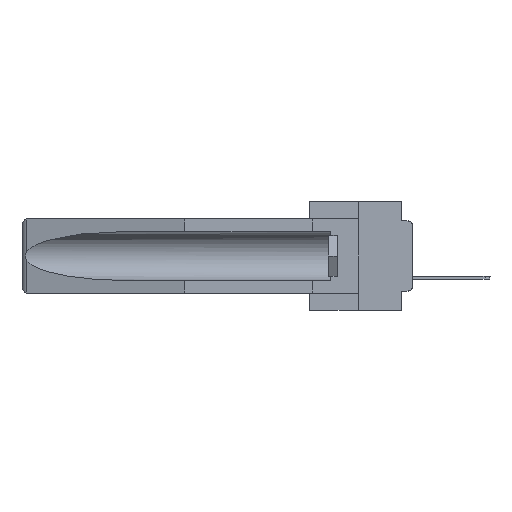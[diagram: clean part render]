
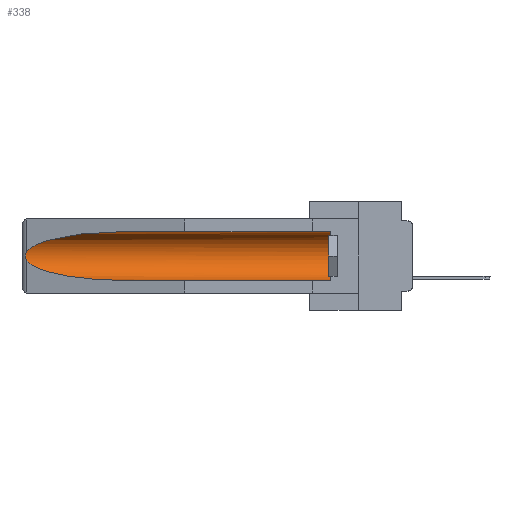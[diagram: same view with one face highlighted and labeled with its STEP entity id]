
A CAD part, left-side view. The second image highlights one B-rep face of the part: STEP entity #338.
In plain terms, the highlighted cylindrical face has radius 2.857 mm (diameter 5.715 mm), a partial arc.
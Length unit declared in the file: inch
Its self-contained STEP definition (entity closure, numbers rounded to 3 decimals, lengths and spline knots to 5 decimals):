
#177 = ORIENTED_EDGE ( 'NONE', *, *, #3073, .T. ) ;
#234 = CARTESIAN_POINT ( 'NONE',  ( 0.155, 1.07973, -0.059 ) ) ;
#338 = ADVANCED_FACE ( 'NONE', ( #30884 ), #16875, .F. ) ;
#2537 = CARTESIAN_POINT ( 'NONE',  ( 0.155, -0.30754, -0.1715 ) ) ;
#3073 = EDGE_CURVE ( 'NONE', #8887, #26737, #36057, .T. ) ;
#3840 = CARTESIAN_POINT ( 'NONE',  ( 0.25451, 1.48313, -0.09465 ) ) ;
#4493 = DIRECTION ( 'NONE',  ( 0., -1., 0. ) ) ;
#5424 = VERTEX_POINT ( 'NONE', #23797 ) ;
#6087 = ORIENTED_EDGE ( 'NONE', *, *, #17450, .T. ) ;
#6566 = CARTESIAN_POINT ( 'NONE',  ( 0.155, -0.30754, -0.284 ) ) ;
#6943 = DIRECTION ( 'NONE',  ( 0., 0., 1. ) ) ;
#6955 = AXIS2_PLACEMENT_3D ( 'NONE', #2537, #21308, #15341 ) ;
#8093 = CARTESIAN_POINT ( 'NONE',  ( 0.25451, 1.48313, -0.24835 ) ) ;
#8133 = AXIS2_PLACEMENT_3D ( 'NONE', #20806, #4493, #6943 ) ;
#8412 = CARTESIAN_POINT ( 'NONE',  ( 0.2673, 1.5327, -0.16383 ) ) ;
#8449 = CARTESIAN_POINT ( 'NONE',  ( 0.155, 1.07973, -0.284 ) ) ;
#8887 = VERTEX_POINT ( 'NONE', #15467 ) ;
#9172 = ORIENTED_EDGE ( 'NONE', *, *, #31409, .T. ) ;
#9975 = VERTEX_POINT ( 'NONE', #25321 ) ;
#10270 = CARTESIAN_POINT ( 'NONE',  ( 0.26597, 1.52961, -0.15275 ) ) ;
#10757 = CIRCLE ( 'NONE', #8133, 0.1125 ) ;
#12735 = ORIENTED_EDGE ( 'NONE', *, *, #32281, .F. ) ;
#14622 = CARTESIAN_POINT ( 'NONE',  ( 0.155, 1.07973, -0.059 ) ) ;
#15341 = DIRECTION ( 'NONE',  ( 0., 0., 1. ) ) ;
#15467 = CARTESIAN_POINT ( 'NONE',  ( 0.26537, 1.52718, -0.14972 ) ) ;
#15515 = CARTESIAN_POINT ( 'NONE',  ( 0.26537, 1.52718, -0.14972 ) ) ;
#15671 = EDGE_CURVE ( 'NONE', #5424, #9975, #10757, .T. ) ;
#16813 = CARTESIAN_POINT ( 'NONE',  ( 0.26537, 1.52718, -0.19328 ) ) ;
#16875 = CYLINDRICAL_SURFACE ( 'NONE', #6955, 0.1125 ) ;
#17039 = CARTESIAN_POINT ( 'NONE',  ( 0.2675, 1.53308, -0.17534 ) ) ;
#17450 = EDGE_CURVE ( 'NONE', #26737, #34620, #21894, .T. ) ;
#19654 =( BOUNDED_CURVE ( )  B_SPLINE_CURVE ( 3, ( #14622, #31401, #3840, #34333 ),
 .UNSPECIFIED., .F., .F. ) 
 B_SPLINE_CURVE_WITH_KNOTS ( ( 4, 4 ),
 ( 4.71239, 6.08839 ),
 .UNSPECIFIED. ) 
 CURVE ( )  GEOMETRIC_REPRESENTATION_ITEM ( )  RATIONAL_B_SPLINE_CURVE ( ( 1., 0.848, 0.848, 1. ) ) 
 REPRESENTATION_ITEM ( '' )  );
#19850 = CARTESIAN_POINT ( 'NONE',  ( 0.2673, 1.53269, -0.17917 ) ) ;
#20299 = DIRECTION ( 'NONE',  ( 0., 1., 0. ) ) ;
#20499 = VERTEX_POINT ( 'NONE', #234 ) ;
#20806 = CARTESIAN_POINT ( 'NONE',  ( 0.155, 0.126, -0.1715 ) ) ;
#21308 = DIRECTION ( 'NONE',  ( 0., 1., 0. ) ) ;
#21894 =( BOUNDED_CURVE ( )  B_SPLINE_CURVE ( 3, ( #27498, #8093, #27612, #30310 ),
 .UNSPECIFIED., .F., .F. ) 
 B_SPLINE_CURVE_WITH_KNOTS ( ( 4, 4 ),
 ( 0.1948, 1.5708 ),
 .UNSPECIFIED. ) 
 CURVE ( )  GEOMETRIC_REPRESENTATION_ITEM ( )  RATIONAL_B_SPLINE_CURVE ( ( 1., 0.848, 0.848, 1. ) ) 
 REPRESENTATION_ITEM ( '' )  );
#22661 = CARTESIAN_POINT ( 'NONE',  ( 0.26655, 1.53094, -0.18657 ) ) ;
#23279 = VECTOR ( 'NONE', #20299, 39.37008 ) ;
#23764 = EDGE_CURVE ( 'NONE', #20499, #8887, #19654, .T. ) ;
#23797 = CARTESIAN_POINT ( 'NONE',  ( 0.155, 0.126, -0.284 ) ) ;
#25036 = DIRECTION ( 'NONE',  ( 0., 1., 0. ) ) ;
#25321 = CARTESIAN_POINT ( 'NONE',  ( 0.155, 0.126, -0.059 ) ) ;
#26737 = VERTEX_POINT ( 'NONE', #16813 ) ;
#27202 = LINE ( 'NONE', #6566, #23279 ) ;
#27498 = CARTESIAN_POINT ( 'NONE',  ( 0.26537, 1.52718, -0.19328 ) ) ;
#27612 = CARTESIAN_POINT ( 'NONE',  ( 0.21114, 1.30732, -0.284 ) ) ;
#27730 = CARTESIAN_POINT ( 'NONE',  ( 0.155, -0.30754, -0.059 ) ) ;
#27951 = CARTESIAN_POINT ( 'NONE',  ( 0.2675, 1.53308, -0.16763 ) ) ;
#28426 = CARTESIAN_POINT ( 'NONE',  ( 0.26597, 1.5296, -0.19026 ) ) ;
#29961 = CARTESIAN_POINT ( 'NONE',  ( 0.26654, 1.53092, -0.15636 ) ) ;
#30310 = CARTESIAN_POINT ( 'NONE',  ( 0.155, 1.07973, -0.284 ) ) ;
#30884 = FACE_OUTER_BOUND ( 'NONE', #35438, .T. ) ;
#31223 = LINE ( 'NONE', #27730, #36073 ) ;
#31401 = CARTESIAN_POINT ( 'NONE',  ( 0.21114, 1.30732, -0.059 ) ) ;
#31409 = EDGE_CURVE ( 'NONE', #9975, #20499, #31223, .T. ) ;
#31856 = ORIENTED_EDGE ( 'NONE', *, *, #23764, .T. ) ;
#32281 = EDGE_CURVE ( 'NONE', #5424, #34620, #27202, .T. ) ;
#34333 = CARTESIAN_POINT ( 'NONE',  ( 0.26537, 1.52718, -0.14972 ) ) ;
#34550 = CARTESIAN_POINT ( 'NONE',  ( 0.26537, 1.52718, -0.19328 ) ) ;
#34620 = VERTEX_POINT ( 'NONE', #8449 ) ;
#34965 = ORIENTED_EDGE ( 'NONE', *, *, #15671, .T. ) ;
#35438 = EDGE_LOOP ( 'NONE', ( #31856, #177, #6087, #12735, #34965, #9172 ) ) ;
#36057 = B_SPLINE_CURVE_WITH_KNOTS ( 'NONE', 3,
 ( #15515, #10270, #29961, #8412, #27951, #17039, #19850, #22661, #28426, #34550 ),
 .UNSPECIFIED., .F., .F.,
 ( 4, 2, 2, 2, 4 ),
 ( 0., 0.00029, 0.00058, 0.00087, 0.00117 ),
 .UNSPECIFIED. ) ;
#36073 = VECTOR ( 'NONE', #25036, 39.37008 ) ;
